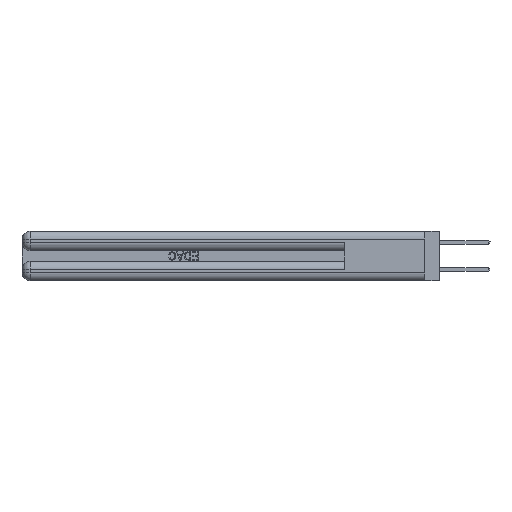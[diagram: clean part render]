
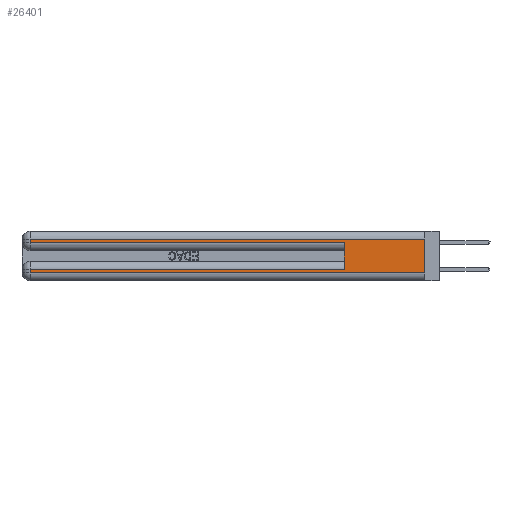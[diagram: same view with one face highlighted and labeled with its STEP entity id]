
A CAD part, left-side view. The second image highlights one B-rep face of the part: STEP entity #26401.
In plain terms, the highlighted planar face has unit normal (-1, 0, 0).
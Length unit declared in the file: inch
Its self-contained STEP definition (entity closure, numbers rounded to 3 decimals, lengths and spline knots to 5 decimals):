
#1763 = EDGE_CURVE ( 'NONE', #36298, #33712, #9771, .T. ) ;
#2210 = AXIS2_PLACEMENT_3D ( 'NONE', #34513, #15298, #42187 ) ;
#2585 = CARTESIAN_POINT ( 'NONE',  ( 0., 0.6, 0.145 ) ) ;
#2705 = ORIENTED_EDGE ( 'NONE', *, *, #42138, .F. ) ;
#3361 = CARTESIAN_POINT ( 'NONE',  ( 0., 0., 0.31 ) ) ;
#3749 = CARTESIAN_POINT ( 'NONE',  ( 0., 2.94, 0.37 ) ) ;
#3925 = VECTOR ( 'NONE', #22022, 39.37008 ) ;
#4525 = LINE ( 'NONE', #38095, #43200 ) ;
#4753 = ORIENTED_EDGE ( 'NONE', *, *, #14878, .F. ) ;
#6128 = CARTESIAN_POINT ( 'NONE',  ( 0., 0., 0.285 ) ) ;
#7673 = DIRECTION ( 'NONE',  ( 0., 0., -1. ) ) ;
#7801 = FACE_OUTER_BOUND ( 'NONE', #38462, .T. ) ;
#9771 = LINE ( 'NONE', #41601, #47126 ) ;
#10120 = ORIENTED_EDGE ( 'NONE', *, *, #44736, .T. ) ;
#10209 = EDGE_CURVE ( 'NONE', #33712, #39951, #34644, .T. ) ;
#10981 = DIRECTION ( 'NONE',  ( 0., 0., -1. ) ) ;
#11363 = PLANE ( 'NONE',  #2210 ) ;
#12158 = VERTEX_POINT ( 'NONE', #41658 ) ;
#12172 = VECTOR ( 'NONE', #33264, 39.37008 ) ;
#14684 = DIRECTION ( 'NONE',  ( 0., 1., 0. ) ) ;
#14878 = EDGE_CURVE ( 'NONE', #36298, #18094, #46219, .T. ) ;
#15298 = DIRECTION ( 'NONE',  ( 1., 0., 0. ) ) ;
#15335 = VECTOR ( 'NONE', #10981, 39.37008 ) ;
#15516 = CARTESIAN_POINT ( 'NONE',  ( 0., 2.94, 0.31 ) ) ;
#17379 = ORIENTED_EDGE ( 'NONE', *, *, #49320, .T. ) ;
#18087 = ORIENTED_EDGE ( 'NONE', *, *, #10209, .T. ) ;
#18094 = VERTEX_POINT ( 'NONE', #35257 ) ;
#18599 = VERTEX_POINT ( 'NONE', #3361 ) ;
#19303 = VECTOR ( 'NONE', #28714, 39.37008 ) ;
#19488 = CARTESIAN_POINT ( 'NONE',  ( 0., 0., 0.37 ) ) ;
#19712 = ORIENTED_EDGE ( 'NONE', *, *, #1763, .T. ) ;
#20070 = CARTESIAN_POINT ( 'NONE',  ( 0., 0.6, 0.085 ) ) ;
#20263 = VERTEX_POINT ( 'NONE', #30556 ) ;
#21028 = LINE ( 'NONE', #3749, #40284 ) ;
#21272 = LINE ( 'NONE', #6128, #12172 ) ;
#22022 = DIRECTION ( 'NONE',  ( 0., 0., 1. ) ) ;
#23408 = DIRECTION ( 'NONE',  ( 0., 0., -1. ) ) ;
#23858 = VERTEX_POINT ( 'NONE', #15516 ) ;
#24063 = CARTESIAN_POINT ( 'NONE',  ( 0., 2.94, 0.085 ) ) ;
#25585 = EDGE_CURVE ( 'NONE', #20263, #18094, #21272, .T. ) ;
#26401 = ADVANCED_FACE ( 'NONE', ( #7801 ), #11363, .F. ) ;
#26682 = DIRECTION ( 'NONE',  ( 0., 1., 0. ) ) ;
#28568 = EDGE_CURVE ( 'NONE', #18599, #23858, #4525, .T. ) ;
#28714 = DIRECTION ( 'NONE',  ( 0., -1., 0. ) ) ;
#29064 = ORIENTED_EDGE ( 'NONE', *, *, #28568, .T. ) ;
#30556 = CARTESIAN_POINT ( 'NONE',  ( 0., 2.94, 0.285 ) ) ;
#33264 = DIRECTION ( 'NONE',  ( 0., -1., 0. ) ) ;
#33712 = VERTEX_POINT ( 'NONE', #24063 ) ;
#34147 = CARTESIAN_POINT ( 'NONE',  ( 0., 2.94, 0.37 ) ) ;
#34513 = CARTESIAN_POINT ( 'NONE',  ( 0., 0., 0.37 ) ) ;
#34587 = LINE ( 'NONE', #19488, #43551 ) ;
#34644 = LINE ( 'NONE', #34147, #15335 ) ;
#35257 = CARTESIAN_POINT ( 'NONE',  ( 0., 0.6, 0.285 ) ) ;
#36298 = VERTEX_POINT ( 'NONE', #20070 ) ;
#38095 = CARTESIAN_POINT ( 'NONE',  ( 0., 0., 0.31 ) ) ;
#38462 = EDGE_LOOP ( 'NONE', ( #2705, #29064, #17379, #45508, #4753, #19712, #18087, #10120 ) ) ;
#39776 = LINE ( 'NONE', #47793, #19303 ) ;
#39951 = VERTEX_POINT ( 'NONE', #48056 ) ;
#40284 = VECTOR ( 'NONE', #7673, 39.37008 ) ;
#41601 = CARTESIAN_POINT ( 'NONE',  ( 0., 0., 0.085 ) ) ;
#41658 = CARTESIAN_POINT ( 'NONE',  ( 0., 0., 0.06 ) ) ;
#42138 = EDGE_CURVE ( 'NONE', #18599, #12158, #34587, .T. ) ;
#42187 = DIRECTION ( 'NONE',  ( 0., 0., -1. ) ) ;
#43200 = VECTOR ( 'NONE', #26682, 39.37008 ) ;
#43551 = VECTOR ( 'NONE', #23408, 39.37008 ) ;
#44736 = EDGE_CURVE ( 'NONE', #39951, #12158, #39776, .T. ) ;
#45508 = ORIENTED_EDGE ( 'NONE', *, *, #25585, .T. ) ;
#46219 = LINE ( 'NONE', #2585, #3925 ) ;
#47126 = VECTOR ( 'NONE', #14684, 39.37008 ) ;
#47793 = CARTESIAN_POINT ( 'NONE',  ( 0., 0., 0.06 ) ) ;
#48056 = CARTESIAN_POINT ( 'NONE',  ( 0., 2.94, 0.06 ) ) ;
#49320 = EDGE_CURVE ( 'NONE', #23858, #20263, #21028, .T. ) ;
